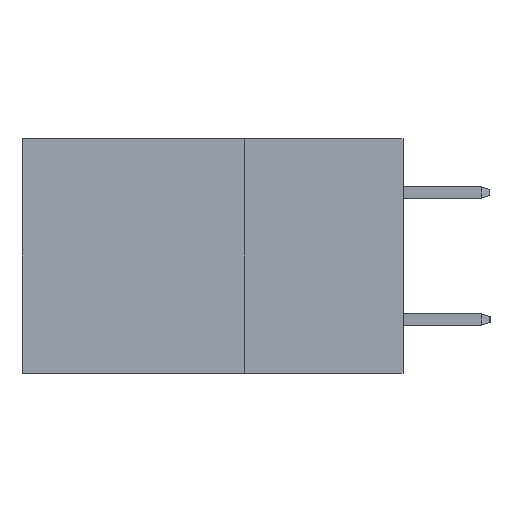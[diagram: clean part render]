
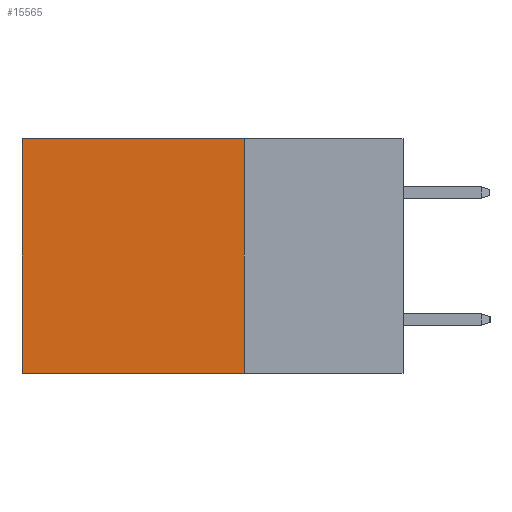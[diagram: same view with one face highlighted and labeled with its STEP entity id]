
A CAD part, left-side view. The second image highlights one B-rep face of the part: STEP entity #15565.
In plain terms, the highlighted planar face has unit normal (-1, 0, 0).
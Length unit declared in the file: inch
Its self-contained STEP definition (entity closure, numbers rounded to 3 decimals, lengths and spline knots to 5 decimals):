
#313 = EDGE_CURVE ( 'NONE', #2751, #13304, #4663, .T. ) ;
#356 = DIRECTION ( 'NONE',  ( 0., 0., -1. ) ) ;
#549 = PLANE ( 'NONE',  #8256 ) ;
#955 = VECTOR ( 'NONE', #10145, 39.37008 ) ;
#1123 = CARTESIAN_POINT ( 'NONE',  ( 0.2875, 0.25, -0.37 ) ) ;
#1618 = CARTESIAN_POINT ( 'NONE',  ( 0.2875, 0.25, 0. ) ) ;
#2751 = VERTEX_POINT ( 'NONE', #8175 ) ;
#3402 = LINE ( 'NONE', #3692, #10792 ) ;
#3499 = FACE_OUTER_BOUND ( 'NONE', #13146, .T. ) ;
#3692 = CARTESIAN_POINT ( 'NONE',  ( 0.2875, 0.25, 0. ) ) ;
#4663 = LINE ( 'NONE', #1618, #4700 ) ;
#4700 = VECTOR ( 'NONE', #6139, 39.37008 ) ;
#4843 = ORIENTED_EDGE ( 'NONE', *, *, #10319, .F. ) ;
#5542 = LINE ( 'NONE', #1123, #955 ) ;
#6038 = CARTESIAN_POINT ( 'NONE',  ( 0.2875, 0.25, -0.37 ) ) ;
#6139 = DIRECTION ( 'NONE',  ( 0., 0., -1. ) ) ;
#6254 = EDGE_CURVE ( 'NONE', #8732, #13892, #7450, .T. ) ;
#7403 = CARTESIAN_POINT ( 'NONE',  ( 0.2875, 0.6, -0.37 ) ) ;
#7450 = LINE ( 'NONE', #17562, #8250 ) ;
#8016 = DIRECTION ( 'NONE',  ( 1., 0., 0. ) ) ;
#8175 = CARTESIAN_POINT ( 'NONE',  ( 0.2875, 0.25, 0. ) ) ;
#8250 = VECTOR ( 'NONE', #10396, 39.37008 ) ;
#8256 = AXIS2_PLACEMENT_3D ( 'NONE', #15401, #8016, #356 ) ;
#8732 = VERTEX_POINT ( 'NONE', #15321 ) ;
#10145 = DIRECTION ( 'NONE',  ( 0., 1., 0. ) ) ;
#10319 = EDGE_CURVE ( 'NONE', #13304, #13892, #5542, .T. ) ;
#10396 = DIRECTION ( 'NONE',  ( 0., 0., -1. ) ) ;
#10792 = VECTOR ( 'NONE', #15488, 39.37008 ) ;
#13146 = EDGE_LOOP ( 'NONE', ( #15447, #4843, #18456, #16403 ) ) ;
#13304 = VERTEX_POINT ( 'NONE', #6038 ) ;
#13892 = VERTEX_POINT ( 'NONE', #7403 ) ;
#15321 = CARTESIAN_POINT ( 'NONE',  ( 0.2875, 0.6, 0. ) ) ;
#15401 = CARTESIAN_POINT ( 'NONE',  ( 0.2875, 0.25, 0. ) ) ;
#15447 = ORIENTED_EDGE ( 'NONE', *, *, #6254, .T. ) ;
#15488 = DIRECTION ( 'NONE',  ( 0., 1., 0. ) ) ;
#15565 = ADVANCED_FACE ( 'NONE', ( #3499 ), #549, .F. ) ;
#15574 = EDGE_CURVE ( 'NONE', #2751, #8732, #3402, .T. ) ;
#16403 = ORIENTED_EDGE ( 'NONE', *, *, #15574, .T. ) ;
#17562 = CARTESIAN_POINT ( 'NONE',  ( 0.2875, 0.6, 0. ) ) ;
#18456 = ORIENTED_EDGE ( 'NONE', *, *, #313, .F. ) ;
